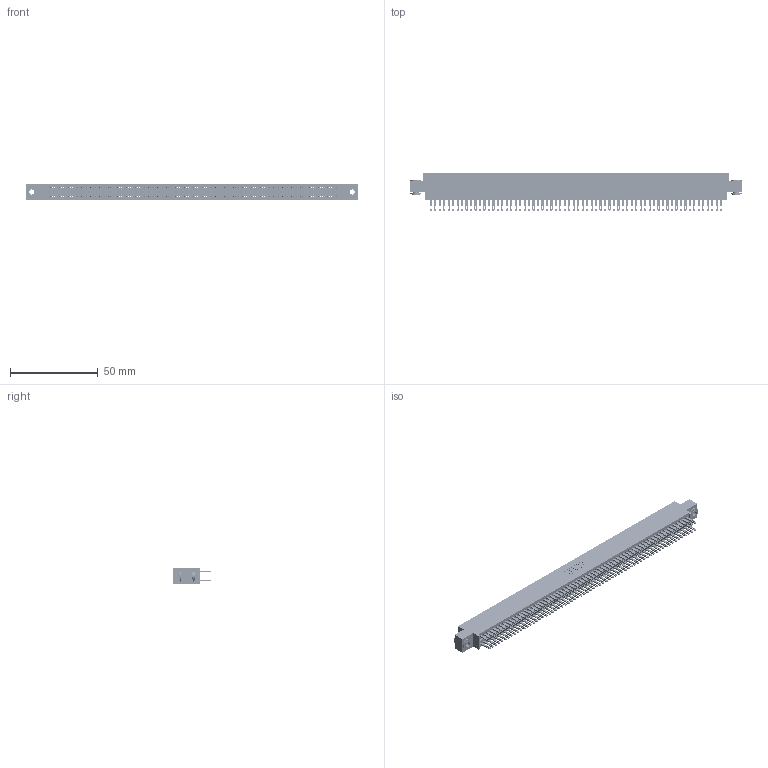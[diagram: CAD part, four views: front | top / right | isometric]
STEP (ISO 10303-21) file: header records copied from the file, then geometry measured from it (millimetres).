
FILE_DESCRIPTION (( 'STEP AP203' ), '1' );
FILE_NAME ('895-132-500-803.STEP', '2020-10-13T17:39:18', ( '' ), ( '' ), 'SwSTEP 2.0', 'SolidWorks 2020', '' );
FILE_SCHEMA (( 'CONFIG_CONTROL_DESIGN' ));
Length unit declared in the file: inch
Products named in the file (4): 845 Part_0.170 Offset - 0.156 Dia-TH; 895-132-500-803; 345-250-002_345-250-002-102; 345-292-001_345-293-100
Assembly tree (135 placements, depth 2):
  895-132-500-803
    845 Part_0.170 Offset - 0.156 Dia-TH
    345-292-001_345-293-100  x132
    345-250-002_345-250-002-102  x2
Bounding box: 188.85 x 21.51 x 9.4 mm (x, y, z)
Volume: 18877.1 mm3; surface area: 30063.1 mm2
Topology: 135 solids, 135 shells, 6240 faces, 19041 edges, 12690 vertices
Faces by surface type: plane 3658, cylinder 2574, cone 8
Entity records: 49266 total; most frequent: CARTESIAN_POINT 8211, ORIENTED_EDGE 8138, DIRECTION 7243, EDGE_CURVE 4069, LINE 3645, VECTOR 3645, VERTEX_POINT 2710, AXIS2_PLACEMENT_3D 1799
